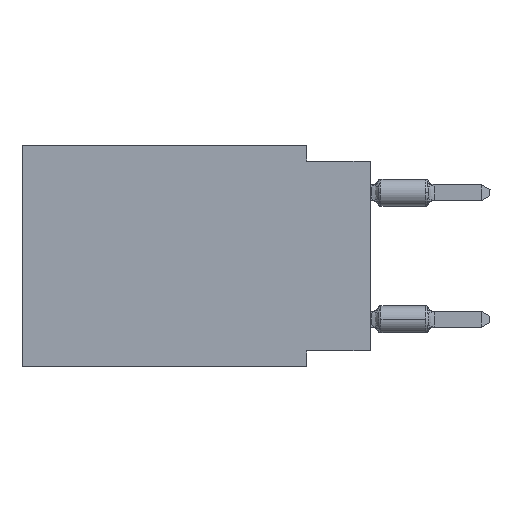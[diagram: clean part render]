
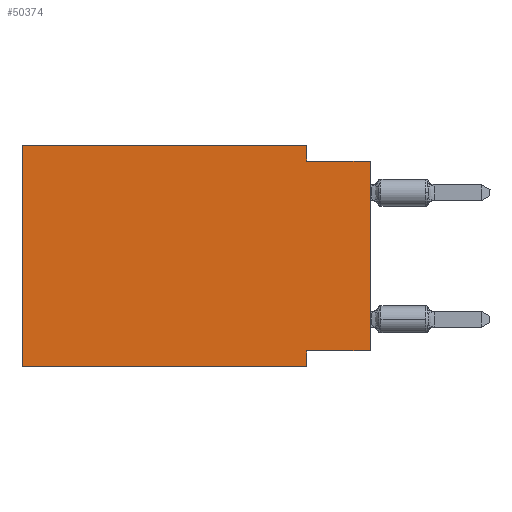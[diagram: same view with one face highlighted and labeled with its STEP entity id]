
A CAD part, left-side view. The second image highlights one B-rep face of the part: STEP entity #50374.
In plain terms, the highlighted planar face has unit normal (-1, 0, 0).
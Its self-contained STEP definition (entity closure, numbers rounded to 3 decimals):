
#2240 = ORIENTED_EDGE ( 'NONE', *, *, #32153, .F. ) ;
#6603 = DIRECTION ( 'NONE',  ( 0., 0., 1. ) ) ;
#7024 = VERTEX_POINT ( 'NONE', #54325 ) ;
#7131 = EDGE_CURVE ( 'NONE', #45025, #38187, #7154, .T. ) ;
#7154 = LINE ( 'NONE', #21682, #37106 ) ;
#7694 = CARTESIAN_POINT ( 'NONE',  ( 0., 13.97, 0. ) ) ;
#7897 = ORIENTED_EDGE ( 'NONE', *, *, #49874, .F. ) ;
#8328 = DIRECTION ( 'NONE',  ( 0., 0., -1. ) ) ;
#8939 = CARTESIAN_POINT ( 'NONE',  ( 0., 0., 0. ) ) ;
#9455 = DIRECTION ( 'NONE',  ( 0., -1., 0. ) ) ;
#9921 = CARTESIAN_POINT ( 'NONE',  ( 0., 2.54, -8.89 ) ) ;
#10332 = EDGE_CURVE ( 'NONE', #61824, #7024, #22239, .T. ) ;
#10977 = VECTOR ( 'NONE', #22245, 1000. ) ;
#11596 = VERTEX_POINT ( 'NONE', #27618 ) ;
#12536 = DIRECTION ( 'NONE',  ( 0., 1., 0. ) ) ;
#12750 = CARTESIAN_POINT ( 'NONE',  ( 0., 2.54, 0. ) ) ;
#13688 = LINE ( 'NONE', #7694, #10977 ) ;
#16029 = VECTOR ( 'NONE', #51603, 1000. ) ;
#16095 = LINE ( 'NONE', #8939, #37475 ) ;
#18858 = DIRECTION ( 'NONE',  ( 0., 0., -1. ) ) ;
#20186 = EDGE_CURVE ( 'NONE', #11596, #38623, #61423, .T. ) ;
#20683 = CARTESIAN_POINT ( 'NONE',  ( 0., 2.54, 0. ) ) ;
#21682 = CARTESIAN_POINT ( 'NONE',  ( 0., 0., -8.255 ) ) ;
#22239 = LINE ( 'NONE', #12750, #26240 ) ;
#22245 = DIRECTION ( 'NONE',  ( 0., 0., 1. ) ) ;
#23389 = ORIENTED_EDGE ( 'NONE', *, *, #10332, .F. ) ;
#23400 = CARTESIAN_POINT ( 'NONE',  ( 0., 13.97, 0. ) ) ;
#23916 = FACE_OUTER_BOUND ( 'NONE', #24814, .T. ) ;
#24300 = CARTESIAN_POINT ( 'NONE',  ( 0., 0., -0.635 ) ) ;
#24814 = EDGE_LOOP ( 'NONE', ( #62431, #36697, #23389, #7897, #2240, #36771, #35237, #47845 ) ) ;
#25027 = VERTEX_POINT ( 'NONE', #32057 ) ;
#26240 = VECTOR ( 'NONE', #8328, 1000. ) ;
#27125 = CARTESIAN_POINT ( 'NONE',  ( 0., 2.54, -8.255 ) ) ;
#27201 = LINE ( 'NONE', #23400, #16029 ) ;
#27618 = CARTESIAN_POINT ( 'NONE',  ( 0., 13.97, -8.89 ) ) ;
#28144 = VECTOR ( 'NONE', #9455, 1000. ) ;
#28175 = CARTESIAN_POINT ( 'NONE',  ( 0., 13.97, -8.89 ) ) ;
#28969 = DIRECTION ( 'NONE',  ( 1., 0., 0. ) ) ;
#32057 = CARTESIAN_POINT ( 'NONE',  ( 0., 13.97, 0. ) ) ;
#32153 = EDGE_CURVE ( 'NONE', #11596, #25027, #13688, .T. ) ;
#35237 = ORIENTED_EDGE ( 'NONE', *, *, #42443, .F. ) ;
#35736 = VECTOR ( 'NONE', #52260, 1000. ) ;
#36697 = ORIENTED_EDGE ( 'NONE', *, *, #49958, .F. ) ;
#36771 = ORIENTED_EDGE ( 'NONE', *, *, #20186, .T. ) ;
#37106 = VECTOR ( 'NONE', #12536, 1000. ) ;
#37475 = VECTOR ( 'NONE', #6603, 1000. ) ;
#38187 = VERTEX_POINT ( 'NONE', #27125 ) ;
#38623 = VERTEX_POINT ( 'NONE', #60938 ) ;
#42443 = EDGE_CURVE ( 'NONE', #38187, #38623, #48251, .T. ) ;
#42930 = EDGE_CURVE ( 'NONE', #45025, #55552, #16095, .T. ) ;
#43227 = CARTESIAN_POINT ( 'NONE',  ( 0., 13.97, 0. ) ) ;
#45025 = VERTEX_POINT ( 'NONE', #58754 ) ;
#47845 = ORIENTED_EDGE ( 'NONE', *, *, #7131, .F. ) ;
#48251 = LINE ( 'NONE', #9921, #53038 ) ;
#49874 = EDGE_CURVE ( 'NONE', #25027, #61824, #27201, .T. ) ;
#49958 = EDGE_CURVE ( 'NONE', #7024, #55552, #58180, .T. ) ;
#50374 = ADVANCED_FACE ( 'NONE', ( #23916 ), #52453, .F. ) ;
#51603 = DIRECTION ( 'NONE',  ( 0., -1., 0. ) ) ;
#52260 = DIRECTION ( 'NONE',  ( 0., -1., 0. ) ) ;
#52453 = PLANE ( 'NONE',  #61587 ) ;
#52698 = DIRECTION ( 'NONE',  ( 0., 0., -1. ) ) ;
#53038 = VECTOR ( 'NONE', #52698, 1000. ) ;
#54325 = CARTESIAN_POINT ( 'NONE',  ( 0., 2.54, -0.635 ) ) ;
#55552 = VERTEX_POINT ( 'NONE', #59969 ) ;
#58180 = LINE ( 'NONE', #24300, #28144 ) ;
#58754 = CARTESIAN_POINT ( 'NONE',  ( 0., 0., -8.255 ) ) ;
#59969 = CARTESIAN_POINT ( 'NONE',  ( 0., 0., -0.635 ) ) ;
#60938 = CARTESIAN_POINT ( 'NONE',  ( 0., 2.54, -8.89 ) ) ;
#61423 = LINE ( 'NONE', #28175, #35736 ) ;
#61587 = AXIS2_PLACEMENT_3D ( 'NONE', #43227, #28969, #18858 ) ;
#61824 = VERTEX_POINT ( 'NONE', #20683 ) ;
#62431 = ORIENTED_EDGE ( 'NONE', *, *, #42930, .T. ) ;
